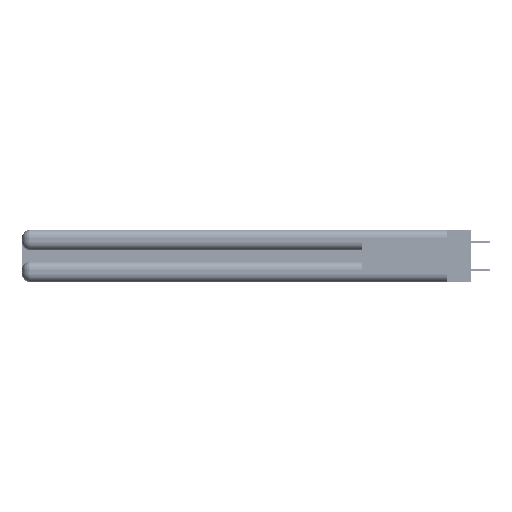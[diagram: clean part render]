
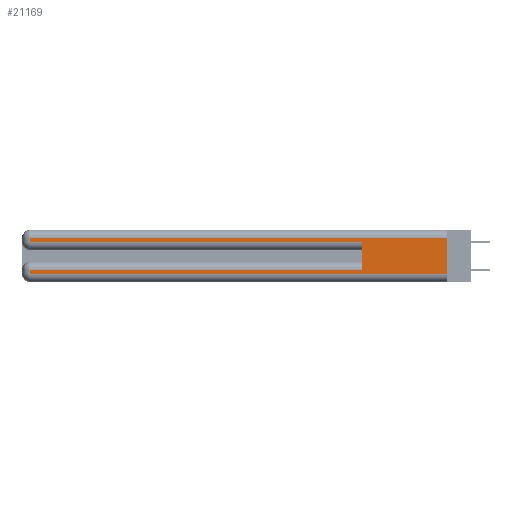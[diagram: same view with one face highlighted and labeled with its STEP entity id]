
A CAD part, left-side view. The second image highlights one B-rep face of the part: STEP entity #21169.
In plain terms, the highlighted planar face has unit normal (-1, 0, 0).
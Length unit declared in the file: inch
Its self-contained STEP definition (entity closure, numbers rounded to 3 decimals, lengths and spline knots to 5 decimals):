
#2424 = LINE ( 'NONE', #16190, #3067 ) ;
#3067 = VECTOR ( 'NONE', #43704, 39.37008 ) ;
#3104 = EDGE_CURVE ( 'NONE', #48822, #18523, #50643, .T. ) ;
#5191 = DIRECTION ( 'NONE',  ( 0., 0., -1. ) ) ;
#6738 = VECTOR ( 'NONE', #32947, 39.37008 ) ;
#7384 = AXIS2_PLACEMENT_3D ( 'NONE', #46061, #51634, #11506 ) ;
#9601 = CARTESIAN_POINT ( 'NONE',  ( 0., 0., 0.06 ) ) ;
#9741 = VECTOR ( 'NONE', #18147, 39.37008 ) ;
#9947 = VERTEX_POINT ( 'NONE', #9601 ) ;
#10759 = DIRECTION ( 'NONE',  ( 0., 1., 0. ) ) ;
#11177 = ORIENTED_EDGE ( 'NONE', *, *, #3104, .F. ) ;
#11506 = DIRECTION ( 'NONE',  ( 0., 0., -1. ) ) ;
#11896 = CARTESIAN_POINT ( 'NONE',  ( 0., 0.6, 0.085 ) ) ;
#14288 = ORIENTED_EDGE ( 'NONE', *, *, #31623, .T. ) ;
#16190 = CARTESIAN_POINT ( 'NONE',  ( 0., 0., 0.37 ) ) ;
#17746 = DIRECTION ( 'NONE',  ( 0., 1., 0. ) ) ;
#18013 = ORIENTED_EDGE ( 'NONE', *, *, #55227, .T. ) ;
#18147 = DIRECTION ( 'NONE',  ( 0., 0., 1. ) ) ;
#18523 = VERTEX_POINT ( 'NONE', #22563 ) ;
#19158 = VECTOR ( 'NONE', #49310, 39.37008 ) ;
#19499 = LINE ( 'NONE', #49965, #6738 ) ;
#19828 = LINE ( 'NONE', #31853, #19978 ) ;
#19978 = VECTOR ( 'NONE', #5191, 39.37008 ) ;
#20451 = VERTEX_POINT ( 'NONE', #44418 ) ;
#20815 = ORIENTED_EDGE ( 'NONE', *, *, #43933, .T. ) ;
#20886 = VECTOR ( 'NONE', #17746, 39.37008 ) ;
#21169 = ADVANCED_FACE ( 'NONE', ( #38419 ), #28185, .F. ) ;
#22155 = VERTEX_POINT ( 'NONE', #29248 ) ;
#22563 = CARTESIAN_POINT ( 'NONE',  ( 0., 0.6, 0.285 ) ) ;
#25081 = CARTESIAN_POINT ( 'NONE',  ( 0., 0., 0.31 ) ) ;
#26568 = VERTEX_POINT ( 'NONE', #46922 ) ;
#26917 = CARTESIAN_POINT ( 'NONE',  ( 0., 0.6, 0.145 ) ) ;
#27299 = CARTESIAN_POINT ( 'NONE',  ( 0., 0., 0.285 ) ) ;
#27359 = VERTEX_POINT ( 'NONE', #45556 ) ;
#27375 = EDGE_CURVE ( 'NONE', #26568, #27359, #19499, .T. ) ;
#28185 = PLANE ( 'NONE',  #7384 ) ;
#29248 = CARTESIAN_POINT ( 'NONE',  ( 0., 0., 0.31 ) ) ;
#29353 = EDGE_CURVE ( 'NONE', #22155, #9947, #2424, .T. ) ;
#29868 = ORIENTED_EDGE ( 'NONE', *, *, #30745, .T. ) ;
#30745 = EDGE_CURVE ( 'NONE', #35410, #20451, #19828, .T. ) ;
#31623 = EDGE_CURVE ( 'NONE', #27359, #18523, #45761, .T. ) ;
#31853 = CARTESIAN_POINT ( 'NONE',  ( 0., 2.94, 0.37 ) ) ;
#32035 = CARTESIAN_POINT ( 'NONE',  ( 0., 0., 0.06 ) ) ;
#32947 = DIRECTION ( 'NONE',  ( 0., 0., -1. ) ) ;
#35410 = VERTEX_POINT ( 'NONE', #36798 ) ;
#36798 = CARTESIAN_POINT ( 'NONE',  ( 0., 2.94, 0.085 ) ) ;
#37935 = VECTOR ( 'NONE', #10759, 39.37008 ) ;
#38419 = FACE_OUTER_BOUND ( 'NONE', #54389, .T. ) ;
#39370 = VECTOR ( 'NONE', #54618, 39.37008 ) ;
#40378 = ORIENTED_EDGE ( 'NONE', *, *, #47829, .T. ) ;
#43021 = ORIENTED_EDGE ( 'NONE', *, *, #29353, .F. ) ;
#43704 = DIRECTION ( 'NONE',  ( 0., 0., -1. ) ) ;
#43933 = EDGE_CURVE ( 'NONE', #22155, #26568, #47353, .T. ) ;
#44418 = CARTESIAN_POINT ( 'NONE',  ( 0., 2.94, 0.06 ) ) ;
#45162 = ORIENTED_EDGE ( 'NONE', *, *, #27375, .T. ) ;
#45556 = CARTESIAN_POINT ( 'NONE',  ( 0., 2.94, 0.285 ) ) ;
#45761 = LINE ( 'NONE', #27299, #19158 ) ;
#46061 = CARTESIAN_POINT ( 'NONE',  ( 0., 0., 0.37 ) ) ;
#46475 = CARTESIAN_POINT ( 'NONE',  ( 0., 0., 0.085 ) ) ;
#46922 = CARTESIAN_POINT ( 'NONE',  ( 0., 2.94, 0.31 ) ) ;
#47353 = LINE ( 'NONE', #25081, #20886 ) ;
#47829 = EDGE_CURVE ( 'NONE', #20451, #9947, #50787, .T. ) ;
#48822 = VERTEX_POINT ( 'NONE', #11896 ) ;
#49310 = DIRECTION ( 'NONE',  ( 0., -1., 0. ) ) ;
#49965 = CARTESIAN_POINT ( 'NONE',  ( 0., 2.94, 0.37 ) ) ;
#50643 = LINE ( 'NONE', #26917, #9741 ) ;
#50787 = LINE ( 'NONE', #32035, #39370 ) ;
#50884 = LINE ( 'NONE', #46475, #37935 ) ;
#51634 = DIRECTION ( 'NONE',  ( 1., 0., 0. ) ) ;
#54389 = EDGE_LOOP ( 'NONE', ( #43021, #20815, #45162, #14288, #11177, #18013, #29868, #40378 ) ) ;
#54618 = DIRECTION ( 'NONE',  ( 0., -1., 0. ) ) ;
#55227 = EDGE_CURVE ( 'NONE', #48822, #35410, #50884, .T. ) ;
